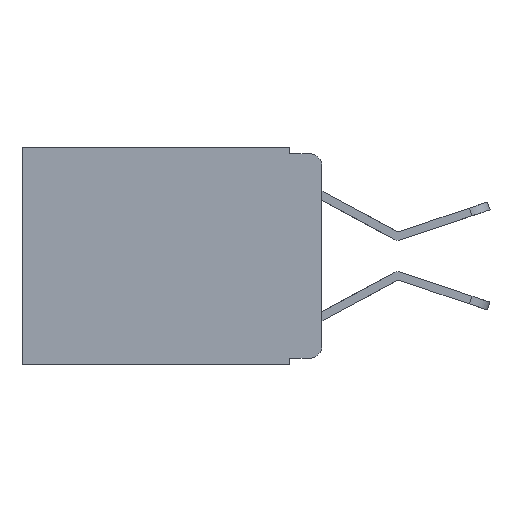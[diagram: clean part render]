
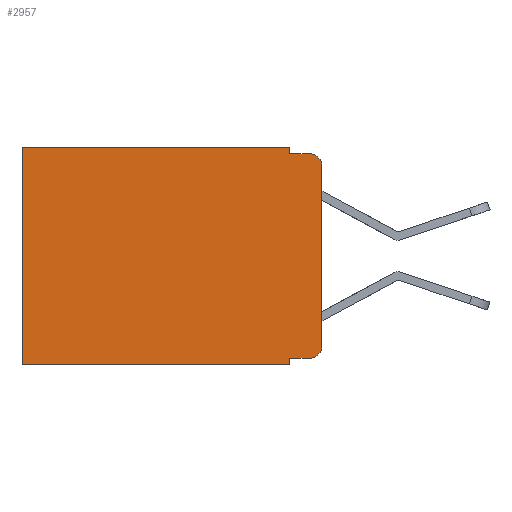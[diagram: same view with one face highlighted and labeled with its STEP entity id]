
A CAD part, left-side view. The second image highlights one B-rep face of the part: STEP entity #2957.
In plain terms, the highlighted planar face has unit normal (-1, 0, 0).
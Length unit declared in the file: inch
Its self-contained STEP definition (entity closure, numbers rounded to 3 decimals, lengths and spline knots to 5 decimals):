
#28 = EDGE_CURVE ( 'NONE', #8597, #7999, #5312, .T. ) ;
#75 = EDGE_CURVE ( 'NONE', #8597, #7646, #4199, .T. ) ;
#258 = VERTEX_POINT ( 'NONE', #5446 ) ;
#282 = EDGE_CURVE ( 'NONE', #3871, #7646, #8779, .T. ) ;
#327 = DIRECTION ( 'NONE',  ( 1., 0., 0. ) ) ;
#498 = EDGE_CURVE ( 'NONE', #9001, #3871, #8362, .T. ) ;
#567 = LINE ( 'NONE', #8716, #3217 ) ;
#876 = CARTESIAN_POINT ( 'NONE',  ( 0.298, 0.051, 0. ) ) ;
#1031 = EDGE_CURVE ( 'NONE', #9001, #258, #5289, .T. ) ;
#1037 = EDGE_CURVE ( 'NONE', #5725, #2257, #10462, .T. ) ;
#1077 = VECTOR ( 'NONE', #9684, 39.37008 ) ;
#1079 = EDGE_CURVE ( 'NONE', #1878, #7999, #9906, .T. ) ;
#1084 = LINE ( 'NONE', #9933, #3648 ) ;
#1196 = EDGE_CURVE ( 'NONE', #3353, #1878, #1084, .T. ) ;
#1746 = CARTESIAN_POINT ( 'NONE',  ( 0.298, 0., -0.343 ) ) ;
#1810 = ORIENTED_EDGE ( 'NONE', *, *, #282, .T. ) ;
#1878 = VERTEX_POINT ( 'NONE', #4700 ) ;
#1898 = CARTESIAN_POINT ( 'NONE',  ( 0.298, 0.051, -0.333 ) ) ;
#2257 = VERTEX_POINT ( 'NONE', #9061 ) ;
#2957 = ADVANCED_FACE ( 'NONE', ( #6891 ), #5648, .F. ) ;
#3023 = ORIENTED_EDGE ( 'NONE', *, *, #1079, .F. ) ;
#3217 = VECTOR ( 'NONE', #3437, 39.37008 ) ;
#3296 = VECTOR ( 'NONE', #4182, 39.37008 ) ;
#3353 = VERTEX_POINT ( 'NONE', #4365 ) ;
#3437 = DIRECTION ( 'NONE',  ( 0., 1., 0. ) ) ;
#3550 = LINE ( 'NONE', #1746, #5485 ) ;
#3596 = CARTESIAN_POINT ( 'NONE',  ( 0.298, 0.02, -0.313 ) ) ;
#3648 = VECTOR ( 'NONE', #6444, 39.37008 ) ;
#3662 = CARTESIAN_POINT ( 'NONE',  ( 0.298, 0.473, 0. ) ) ;
#3854 = EDGE_LOOP ( 'NONE', ( #3896, #5332, #3023, #6433, #6647, #9552, #8072, #9374, #8785, #1810 ) ) ;
#3871 = VERTEX_POINT ( 'NONE', #4465 ) ;
#3896 = ORIENTED_EDGE ( 'NONE', *, *, #75, .F. ) ;
#4182 = DIRECTION ( 'NONE',  ( 0., 0., -1. ) ) ;
#4199 = LINE ( 'NONE', #4216, #1077 ) ;
#4216 = CARTESIAN_POINT ( 'NONE',  ( 0.298, 0., 0. ) ) ;
#4365 = CARTESIAN_POINT ( 'NONE',  ( 0.298, 0.051, 0. ) ) ;
#4420 = AXIS2_PLACEMENT_3D ( 'NONE', #7586, #6750, #10022 ) ;
#4465 = CARTESIAN_POINT ( 'NONE',  ( 0.298, 0.02, -0.333 ) ) ;
#4700 = CARTESIAN_POINT ( 'NONE',  ( 0.298, 0.051, -0.01 ) ) ;
#5050 = DIRECTION ( 'NONE',  ( -1., 0., 0. ) ) ;
#5289 = LINE ( 'NONE', #876, #3296 ) ;
#5312 = CIRCLE ( 'NONE', #4420, 0.02 ) ;
#5332 = ORIENTED_EDGE ( 'NONE', *, *, #28, .T. ) ;
#5446 = CARTESIAN_POINT ( 'NONE',  ( 0.298, 0.051, -0.343 ) ) ;
#5485 = VECTOR ( 'NONE', #9638, 39.37008 ) ;
#5530 = CARTESIAN_POINT ( 'NONE',  ( 0.298, 0.051, -0.333 ) ) ;
#5648 = PLANE ( 'NONE',  #9810 ) ;
#5725 = VERTEX_POINT ( 'NONE', #3662 ) ;
#6016 = DIRECTION ( 'NONE',  ( 0., 0., -1. ) ) ;
#6433 = ORIENTED_EDGE ( 'NONE', *, *, #1196, .F. ) ;
#6444 = DIRECTION ( 'NONE',  ( 0., 0., -1. ) ) ;
#6522 = VECTOR ( 'NONE', #6701, 39.37008 ) ;
#6561 = CARTESIAN_POINT ( 'NONE',  ( 0.298, 0., -0.313 ) ) ;
#6647 = ORIENTED_EDGE ( 'NONE', *, *, #9510, .T. ) ;
#6701 = DIRECTION ( 'NONE',  ( 0., -1., 0. ) ) ;
#6750 = DIRECTION ( 'NONE',  ( -1., 0., 0. ) ) ;
#6891 = FACE_OUTER_BOUND ( 'NONE', #3854, .T. ) ;
#7128 = EDGE_CURVE ( 'NONE', #258, #2257, #3550, .T. ) ;
#7586 = CARTESIAN_POINT ( 'NONE',  ( 0.298, 0.02, -0.03 ) ) ;
#7646 = VERTEX_POINT ( 'NONE', #6561 ) ;
#7783 = DIRECTION ( 'NONE',  ( 0., -1., 0. ) ) ;
#7867 = DIRECTION ( 'NONE',  ( 0., 0., -1. ) ) ;
#7909 = AXIS2_PLACEMENT_3D ( 'NONE', #3596, #5050, #6016 ) ;
#7999 = VERTEX_POINT ( 'NONE', #8750 ) ;
#8072 = ORIENTED_EDGE ( 'NONE', *, *, #7128, .F. ) ;
#8256 = CARTESIAN_POINT ( 'NONE',  ( 0.298, 0.473, 0. ) ) ;
#8284 = CARTESIAN_POINT ( 'NONE',  ( 0.298, 0.051, -0.01 ) ) ;
#8362 = LINE ( 'NONE', #5530, #6522 ) ;
#8597 = VERTEX_POINT ( 'NONE', #8978 ) ;
#8716 = CARTESIAN_POINT ( 'NONE',  ( 0.298, 0., 0. ) ) ;
#8750 = CARTESIAN_POINT ( 'NONE',  ( 0.298, 0.02, -0.01 ) ) ;
#8779 = CIRCLE ( 'NONE', #7909, 0.02 ) ;
#8785 = ORIENTED_EDGE ( 'NONE', *, *, #498, .T. ) ;
#8860 = VECTOR ( 'NONE', #7867, 39.37008 ) ;
#8978 = CARTESIAN_POINT ( 'NONE',  ( 0.298, 0., -0.03 ) ) ;
#9001 = VERTEX_POINT ( 'NONE', #1898 ) ;
#9061 = CARTESIAN_POINT ( 'NONE',  ( 0.298, 0.473, -0.343 ) ) ;
#9250 = DIRECTION ( 'NONE',  ( 0., 0., -1. ) ) ;
#9374 = ORIENTED_EDGE ( 'NONE', *, *, #1031, .F. ) ;
#9425 = CARTESIAN_POINT ( 'NONE',  ( 0.298, 0., 0. ) ) ;
#9510 = EDGE_CURVE ( 'NONE', #3353, #5725, #567, .T. ) ;
#9552 = ORIENTED_EDGE ( 'NONE', *, *, #1037, .T. ) ;
#9638 = DIRECTION ( 'NONE',  ( 0., 1., 0. ) ) ;
#9684 = DIRECTION ( 'NONE',  ( 0., 0., -1. ) ) ;
#9719 = VECTOR ( 'NONE', #7783, 39.37008 ) ;
#9810 = AXIS2_PLACEMENT_3D ( 'NONE', #9425, #327, #9250 ) ;
#9906 = LINE ( 'NONE', #8284, #9719 ) ;
#9933 = CARTESIAN_POINT ( 'NONE',  ( 0.298, 0.051, 0. ) ) ;
#10022 = DIRECTION ( 'NONE',  ( 0., 0., -1. ) ) ;
#10462 = LINE ( 'NONE', #8256, #8860 ) ;
